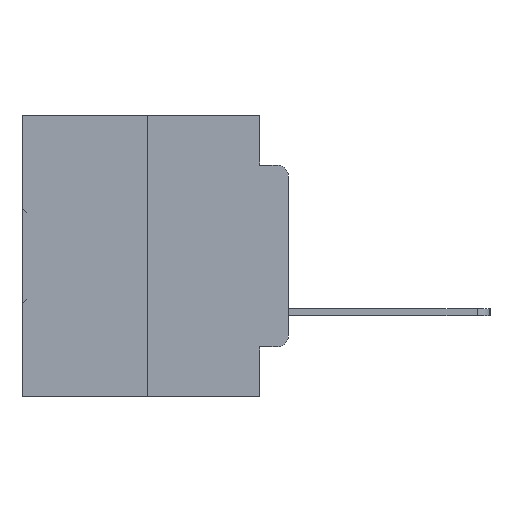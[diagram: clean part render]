
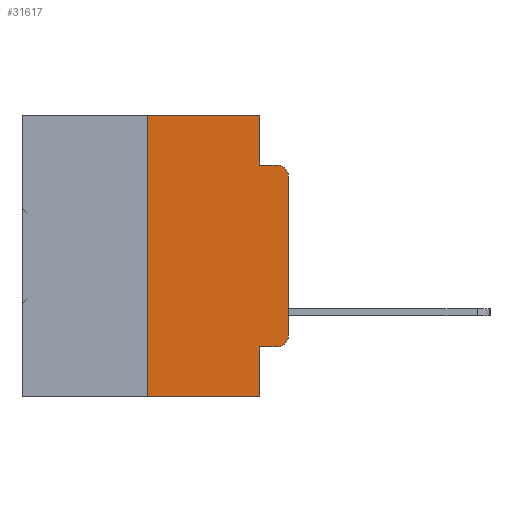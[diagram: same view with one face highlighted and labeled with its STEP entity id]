
A CAD part, left-side view. The second image highlights one B-rep face of the part: STEP entity #31617.
In plain terms, the highlighted planar face has unit normal (-1, 0, 0).
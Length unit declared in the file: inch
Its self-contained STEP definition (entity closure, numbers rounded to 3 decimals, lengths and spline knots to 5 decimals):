
#150 = CARTESIAN_POINT ( 'NONE',  ( 0., 0.051, -0.5 ) ) ;
#417 = LINE ( 'NONE', #14118, #13924 ) ;
#1562 = VECTOR ( 'NONE', #9796, 39.37008 ) ;
#1852 = EDGE_CURVE ( 'NONE', #23369, #26521, #7398, .T. ) ;
#2111 = CIRCLE ( 'NONE', #16084, 0.02 ) ;
#2117 = EDGE_LOOP ( 'NONE', ( #8452, #4959, #18743, #14228, #30604, #22000, #12179, #30565, #24092, #17066 ) ) ;
#2783 = DIRECTION ( 'NONE',  ( 0., 0., -1. ) ) ;
#2889 = DIRECTION ( 'NONE',  ( 0., 0., 1. ) ) ;
#4081 = CARTESIAN_POINT ( 'NONE',  ( 0., 0., -0.3915 ) ) ;
#4959 = ORIENTED_EDGE ( 'NONE', *, *, #32475, .T. ) ;
#5242 = CARTESIAN_POINT ( 'NONE',  ( 0., 0.051, -0.0885 ) ) ;
#5352 = CARTESIAN_POINT ( 'NONE',  ( 0., 0.02, -0.4115 ) ) ;
#6100 = CARTESIAN_POINT ( 'NONE',  ( 0., 0.051, -0.4115 ) ) ;
#6856 = CARTESIAN_POINT ( 'NONE',  ( 0., 0.25, -0.5 ) ) ;
#7137 = DIRECTION ( 'NONE',  ( -1., 0., 0. ) ) ;
#7398 = LINE ( 'NONE', #9486, #14447 ) ;
#8452 = ORIENTED_EDGE ( 'NONE', *, *, #29031, .T. ) ;
#8868 = CARTESIAN_POINT ( 'NONE',  ( 0., 0., 0. ) ) ;
#9486 = CARTESIAN_POINT ( 'NONE',  ( 0., 0.473, 0. ) ) ;
#9701 = EDGE_CURVE ( 'NONE', #29463, #26204, #25452, .T. ) ;
#9796 = DIRECTION ( 'NONE',  ( 0., -1., 0. ) ) ;
#9896 = CARTESIAN_POINT ( 'NONE',  ( 0., 0.02, -0.1085 ) ) ;
#11014 = VERTEX_POINT ( 'NONE', #6100 ) ;
#11083 = CARTESIAN_POINT ( 'NONE',  ( 0., 0.051, 0. ) ) ;
#11360 = LINE ( 'NONE', #33000, #25353 ) ;
#12179 = ORIENTED_EDGE ( 'NONE', *, *, #33916, .T. ) ;
#12518 = DIRECTION ( 'NONE',  ( 0., 0., -1. ) ) ;
#12688 = VERTEX_POINT ( 'NONE', #5242 ) ;
#12689 = VECTOR ( 'NONE', #29156, 39.37008 ) ;
#13232 = EDGE_CURVE ( 'NONE', #11014, #29463, #32702, .T. ) ;
#13451 = CARTESIAN_POINT ( 'NONE',  ( 0., 0.051, -0.4115 ) ) ;
#13592 = LINE ( 'NONE', #17416, #33580 ) ;
#13924 = VECTOR ( 'NONE', #16731, 39.37008 ) ;
#14118 = CARTESIAN_POINT ( 'NONE',  ( 0., 0.051, 0. ) ) ;
#14228 = ORIENTED_EDGE ( 'NONE', *, *, #27290, .F. ) ;
#14447 = VECTOR ( 'NONE', #23799, 39.37008 ) ;
#14515 = AXIS2_PLACEMENT_3D ( 'NONE', #16111, #18762, #2783 ) ;
#14802 = CARTESIAN_POINT ( 'NONE',  ( 0., 0., -0.1085 ) ) ;
#15115 = AXIS2_PLACEMENT_3D ( 'NONE', #22946, #7137, #25629 ) ;
#15318 = VERTEX_POINT ( 'NONE', #14802 ) ;
#15828 = LINE ( 'NONE', #25561, #1562 ) ;
#16084 = AXIS2_PLACEMENT_3D ( 'NONE', #9896, #28217, #12518 ) ;
#16111 = CARTESIAN_POINT ( 'NONE',  ( 0., 0.473, 0. ) ) ;
#16428 = FACE_OUTER_BOUND ( 'NONE', #2117, .T. ) ;
#16556 = VERTEX_POINT ( 'NONE', #29759 ) ;
#16731 = DIRECTION ( 'NONE',  ( 0., 0., -1. ) ) ;
#17066 = ORIENTED_EDGE ( 'NONE', *, *, #9701, .T. ) ;
#17378 = DIRECTION ( 'NONE',  ( 0., 0., -1. ) ) ;
#17416 = CARTESIAN_POINT ( 'NONE',  ( 0., 0.051, -0.0885 ) ) ;
#18498 = EDGE_CURVE ( 'NONE', #11014, #18626, #11360, .T. ) ;
#18626 = VERTEX_POINT ( 'NONE', #150 ) ;
#18743 = ORIENTED_EDGE ( 'NONE', *, *, #25575, .F. ) ;
#18762 = DIRECTION ( 'NONE',  ( 1., 0., 0. ) ) ;
#22000 = ORIENTED_EDGE ( 'NONE', *, *, #22017, .F. ) ;
#22017 = EDGE_CURVE ( 'NONE', #26177, #23369, #29536, .T. ) ;
#22550 = VECTOR ( 'NONE', #2889, 39.37008 ) ;
#22946 = CARTESIAN_POINT ( 'NONE',  ( 0., 0.02, -0.3915 ) ) ;
#23369 = VERTEX_POINT ( 'NONE', #27474 ) ;
#23799 = DIRECTION ( 'NONE',  ( 0., -1., 0. ) ) ;
#24092 = ORIENTED_EDGE ( 'NONE', *, *, #13232, .T. ) ;
#24325 = LINE ( 'NONE', #8868, #29617 ) ;
#25353 = VECTOR ( 'NONE', #17378, 39.37008 ) ;
#25452 = CIRCLE ( 'NONE', #15115, 0.02 ) ;
#25561 = CARTESIAN_POINT ( 'NONE',  ( 0., 0.473, -0.5 ) ) ;
#25575 = EDGE_CURVE ( 'NONE', #12688, #16556, #13592, .T. ) ;
#25629 = DIRECTION ( 'NONE',  ( 0., 0., -1. ) ) ;
#26177 = VERTEX_POINT ( 'NONE', #6856 ) ;
#26204 = VERTEX_POINT ( 'NONE', #4081 ) ;
#26521 = VERTEX_POINT ( 'NONE', #11083 ) ;
#27290 = EDGE_CURVE ( 'NONE', #26521, #12688, #417, .T. ) ;
#27474 = CARTESIAN_POINT ( 'NONE',  ( 0., 0.25, 0. ) ) ;
#28217 = DIRECTION ( 'NONE',  ( -1., 0., 0. ) ) ;
#29031 = EDGE_CURVE ( 'NONE', #26204, #15318, #24325, .T. ) ;
#29156 = DIRECTION ( 'NONE',  ( 0., -1., 0. ) ) ;
#29463 = VERTEX_POINT ( 'NONE', #5352 ) ;
#29536 = LINE ( 'NONE', #31878, #22550 ) ;
#29617 = VECTOR ( 'NONE', #29851, 39.37008 ) ;
#29759 = CARTESIAN_POINT ( 'NONE',  ( 0., 0.02, -0.0885 ) ) ;
#29851 = DIRECTION ( 'NONE',  ( 0., 0., 1. ) ) ;
#30565 = ORIENTED_EDGE ( 'NONE', *, *, #18498, .F. ) ;
#30604 = ORIENTED_EDGE ( 'NONE', *, *, #1852, .F. ) ;
#31617 = ADVANCED_FACE ( 'NONE', ( #16428 ), #31764, .F. ) ;
#31764 = PLANE ( 'NONE',  #14515 ) ;
#31878 = CARTESIAN_POINT ( 'NONE',  ( 0., 0.25, 0. ) ) ;
#32475 = EDGE_CURVE ( 'NONE', #15318, #16556, #2111, .T. ) ;
#32702 = LINE ( 'NONE', #13451, #12689 ) ;
#33000 = CARTESIAN_POINT ( 'NONE',  ( 0., 0.051, 0. ) ) ;
#33042 = DIRECTION ( 'NONE',  ( 0., -1., 0. ) ) ;
#33580 = VECTOR ( 'NONE', #33042, 39.37008 ) ;
#33916 = EDGE_CURVE ( 'NONE', #26177, #18626, #15828, .T. ) ;
